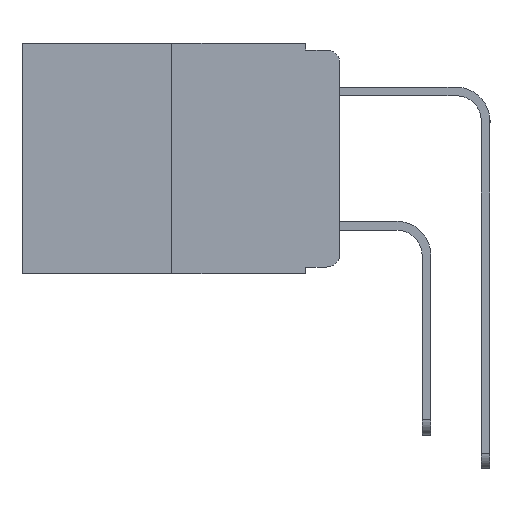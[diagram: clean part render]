
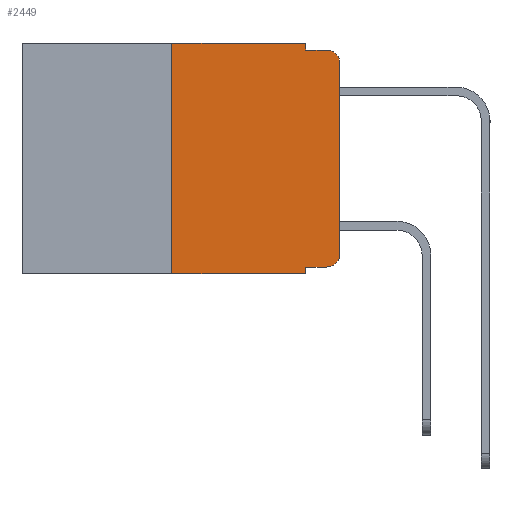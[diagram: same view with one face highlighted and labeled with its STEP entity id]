
A CAD part, left-side view. The second image highlights one B-rep face of the part: STEP entity #2449.
In plain terms, the highlighted planar face has unit normal (-1, 0, 0).
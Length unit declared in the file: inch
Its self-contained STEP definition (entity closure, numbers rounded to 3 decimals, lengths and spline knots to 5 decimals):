
#16 = ORIENTED_EDGE ( 'NONE', *, *, #10471, .F. ) ;
#77 = VECTOR ( 'NONE', #11161, 39.37008 ) ;
#254 = ORIENTED_EDGE ( 'NONE', *, *, #11338, .F. ) ;
#284 = CARTESIAN_POINT ( 'NONE',  ( 0., 0., -0.03 ) ) ;
#358 = ORIENTED_EDGE ( 'NONE', *, *, #4001, .F. ) ;
#702 = VECTOR ( 'NONE', #12523, 39.37008 ) ;
#1032 = LINE ( 'NONE', #14603, #3915 ) ;
#1140 = DIRECTION ( 'NONE',  ( 0., 0., 1. ) ) ;
#1148 = ORIENTED_EDGE ( 'NONE', *, *, #8457, .F. ) ;
#1226 = VERTEX_POINT ( 'NONE', #8204 ) ;
#1336 = CARTESIAN_POINT ( 'NONE',  ( 0., 0.25, 0. ) ) ;
#1379 = ORIENTED_EDGE ( 'NONE', *, *, #11295, .T. ) ;
#1566 = VERTEX_POINT ( 'NONE', #10416 ) ;
#1880 = CARTESIAN_POINT ( 'NONE',  ( 0., 0., -0.313 ) ) ;
#2085 = VERTEX_POINT ( 'NONE', #1880 ) ;
#2449 = ADVANCED_FACE ( 'NONE', ( #11510 ), #11839, .F. ) ;
#2776 = CIRCLE ( 'NONE', #8931, 0.02 ) ;
#3282 = LINE ( 'NONE', #8014, #11888 ) ;
#3316 = DIRECTION ( 'NONE',  ( 0., -1., 0. ) ) ;
#3627 = VERTEX_POINT ( 'NONE', #11123 ) ;
#3841 = EDGE_CURVE ( 'NONE', #11608, #1566, #11477, .T. ) ;
#3915 = VECTOR ( 'NONE', #1140, 39.37008 ) ;
#4001 = EDGE_CURVE ( 'NONE', #13932, #6173, #12320, .T. ) ;
#4654 = VERTEX_POINT ( 'NONE', #14632 ) ;
#4945 = ORIENTED_EDGE ( 'NONE', *, *, #9232, .T. ) ;
#4955 = EDGE_CURVE ( 'NONE', #1226, #3627, #7077, .T. ) ;
#5063 = EDGE_LOOP ( 'NONE', ( #6677, #9410, #16, #254, #358, #1148, #1379, #12306, #5328, #4945 ) ) ;
#5328 = ORIENTED_EDGE ( 'NONE', *, *, #6527, .T. ) ;
#5424 = DIRECTION ( 'NONE',  ( -1., 0., 0. ) ) ;
#5998 = CARTESIAN_POINT ( 'NONE',  ( 0., 0.02, -0.313 ) ) ;
#6173 = VERTEX_POINT ( 'NONE', #7636 ) ;
#6527 = EDGE_CURVE ( 'NONE', #1226, #4654, #13222, .T. ) ;
#6677 = ORIENTED_EDGE ( 'NONE', *, *, #12610, .T. ) ;
#6889 = DIRECTION ( 'NONE',  ( 0., -1., 0. ) ) ;
#6962 = CARTESIAN_POINT ( 'NONE',  ( 0., 0.051, -0.01 ) ) ;
#7077 = LINE ( 'NONE', #9408, #702 ) ;
#7146 = DIRECTION ( 'NONE',  ( 0., 0., -1. ) ) ;
#7479 = VECTOR ( 'NONE', #6889, 39.37008 ) ;
#7542 = CARTESIAN_POINT ( 'NONE',  ( 0., 0.473, 0. ) ) ;
#7636 = CARTESIAN_POINT ( 'NONE',  ( 0., 0.051, 0. ) ) ;
#8014 = CARTESIAN_POINT ( 'NONE',  ( 0., 0.473, -0.343 ) ) ;
#8178 = CARTESIAN_POINT ( 'NONE',  ( 0., 0.473, 0. ) ) ;
#8204 = CARTESIAN_POINT ( 'NONE',  ( 0., 0.051, -0.333 ) ) ;
#8457 = EDGE_CURVE ( 'NONE', #13971, #13932, #10811, .T. ) ;
#8488 = DIRECTION ( 'NONE',  ( 0., 0., -1. ) ) ;
#8650 = VERTEX_POINT ( 'NONE', #6962 ) ;
#8854 = DIRECTION ( 'NONE',  ( 1., 0., 0. ) ) ;
#8931 = AXIS2_PLACEMENT_3D ( 'NONE', #5998, #13626, #7146 ) ;
#9064 = VECTOR ( 'NONE', #13596, 39.37008 ) ;
#9232 = EDGE_CURVE ( 'NONE', #4654, #2085, #2776, .T. ) ;
#9408 = CARTESIAN_POINT ( 'NONE',  ( 0., 0.051, 0. ) ) ;
#9410 = ORIENTED_EDGE ( 'NONE', *, *, #3841, .T. ) ;
#9755 = LINE ( 'NONE', #12494, #9064 ) ;
#9923 = AXIS2_PLACEMENT_3D ( 'NONE', #7542, #8854, #8488 ) ;
#10416 = CARTESIAN_POINT ( 'NONE',  ( 0., 0.02, -0.01 ) ) ;
#10471 = EDGE_CURVE ( 'NONE', #8650, #1566, #9755, .T. ) ;
#10811 = LINE ( 'NONE', #13130, #13328 ) ;
#11123 = CARTESIAN_POINT ( 'NONE',  ( 0., 0.051, -0.343 ) ) ;
#11136 = CARTESIAN_POINT ( 'NONE',  ( 0., 0.051, -0.333 ) ) ;
#11161 = DIRECTION ( 'NONE',  ( 0., -1., 0. ) ) ;
#11295 = EDGE_CURVE ( 'NONE', #13971, #3627, #3282, .T. ) ;
#11338 = EDGE_CURVE ( 'NONE', #6173, #8650, #11551, .T. ) ;
#11477 = CIRCLE ( 'NONE', #11690, 0.02 ) ;
#11510 = FACE_OUTER_BOUND ( 'NONE', #5063, .T. ) ;
#11551 = LINE ( 'NONE', #13478, #14092 ) ;
#11608 = VERTEX_POINT ( 'NONE', #284 ) ;
#11690 = AXIS2_PLACEMENT_3D ( 'NONE', #13235, #5424, #14190 ) ;
#11839 = PLANE ( 'NONE',  #9923 ) ;
#11888 = VECTOR ( 'NONE', #3316, 39.37008 ) ;
#12306 = ORIENTED_EDGE ( 'NONE', *, *, #4955, .F. ) ;
#12320 = LINE ( 'NONE', #8178, #77 ) ;
#12494 = CARTESIAN_POINT ( 'NONE',  ( 0., 0.051, -0.01 ) ) ;
#12523 = DIRECTION ( 'NONE',  ( 0., 0., -1. ) ) ;
#12610 = EDGE_CURVE ( 'NONE', #2085, #11608, #1032, .T. ) ;
#13130 = CARTESIAN_POINT ( 'NONE',  ( 0., 0.25, 0. ) ) ;
#13222 = LINE ( 'NONE', #11136, #7479 ) ;
#13235 = CARTESIAN_POINT ( 'NONE',  ( 0., 0.02, -0.03 ) ) ;
#13328 = VECTOR ( 'NONE', #14195, 39.37008 ) ;
#13478 = CARTESIAN_POINT ( 'NONE',  ( 0., 0.051, 0. ) ) ;
#13596 = DIRECTION ( 'NONE',  ( 0., -1., 0. ) ) ;
#13626 = DIRECTION ( 'NONE',  ( -1., 0., 0. ) ) ;
#13792 = CARTESIAN_POINT ( 'NONE',  ( 0., 0.25, -0.343 ) ) ;
#13932 = VERTEX_POINT ( 'NONE', #1336 ) ;
#13971 = VERTEX_POINT ( 'NONE', #13792 ) ;
#14092 = VECTOR ( 'NONE', #14536, 39.37008 ) ;
#14190 = DIRECTION ( 'NONE',  ( 0., 0., -1. ) ) ;
#14195 = DIRECTION ( 'NONE',  ( 0., 0., 1. ) ) ;
#14536 = DIRECTION ( 'NONE',  ( 0., 0., -1. ) ) ;
#14603 = CARTESIAN_POINT ( 'NONE',  ( 0., 0., 0. ) ) ;
#14632 = CARTESIAN_POINT ( 'NONE',  ( 0., 0.02, -0.333 ) ) ;
